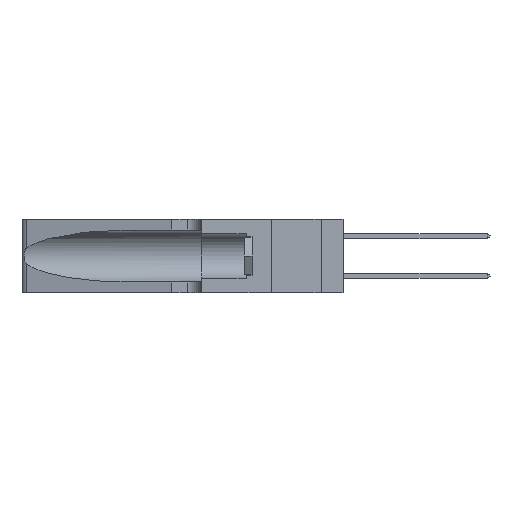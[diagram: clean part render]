
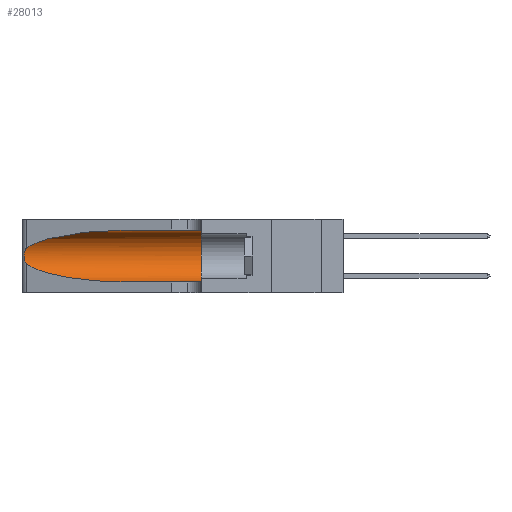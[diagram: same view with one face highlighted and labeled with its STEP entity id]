
A CAD part, left-side view. The second image highlights one B-rep face of the part: STEP entity #28013.
In plain terms, the highlighted cylindrical face has radius 3.308 mm (diameter 6.617 mm), a partial arc.
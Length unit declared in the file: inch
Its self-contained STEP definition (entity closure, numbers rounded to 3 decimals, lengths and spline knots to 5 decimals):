
#262 = VERTEX_POINT ( 'NONE', #25707 ) ;
#664 = CARTESIAN_POINT ( 'NONE',  ( 0.26075, 1.23896, 0.178 ) ) ;
#1474 = DIRECTION ( 'NONE',  ( 0., 0., 1. ) ) ;
#3393 = CARTESIAN_POINT ( 'NONE',  ( 0.25487, 1.22718, 0.14631 ) ) ;
#3429 = CARTESIAN_POINT ( 'NONE',  ( 0.25856, 1.23593, 0.16098 ) ) ;
#3610 = CARTESIAN_POINT ( 'NONE',  ( 0.1305, 0.35, 0.05475 ) ) ;
#3650 = DIRECTION ( 'NONE',  ( 0., -1., 0. ) ) ;
#3895 = CYLINDRICAL_SURFACE ( 'NONE', #28945, 0.13025 ) ;
#4145 = LINE ( 'NONE', #28352, #26777 ) ;
#4818 = CIRCLE ( 'NONE', #6387, 0.13025 ) ;
#5707 = VERTEX_POINT ( 'NONE', #3610 ) ;
#6070 = B_SPLINE_CURVE_WITH_KNOTS ( 'NONE', 3,
 ( #11568, #19654, #22416, #30575, #14310, #33290, #17061, #664, #19772, #3429, #22539, #6186, #25286, #8914 ),
 .UNSPECIFIED., .F., .F.,
 ( 4, 2, 2, 2, 2, 2, 4 ),
 ( 0., 0.00027, 0.00053, 0.00107, 0.0016, 0.00187, 0.00214 ),
 .UNSPECIFIED. ) ;
#6186 = CARTESIAN_POINT ( 'NONE',  ( 0.25639, 1.23186, 0.15144 ) ) ;
#6387 = AXIS2_PLACEMENT_3D ( 'NONE', #34087, #17839, #1474 ) ;
#7139 =( BOUNDED_CURVE ( )  B_SPLINE_CURVE ( 3, ( #25425, #30601, #30829, #14572 ),
 .UNSPECIFIED., .F., .F. ) 
 B_SPLINE_CURVE_WITH_KNOTS ( ( 4, 4 ),
 ( 1.5708, 2.84003 ),
 .UNSPECIFIED. ) 
 CURVE ( )  GEOMETRIC_REPRESENTATION_ITEM ( )  RATIONAL_B_SPLINE_CURVE ( ( 1., 0.87, 0.87, 1. ) ) 
 REPRESENTATION_ITEM ( '' )  );
#8318 = ORIENTED_EDGE ( 'NONE', *, *, #19628, .T. ) ;
#8880 = CARTESIAN_POINT ( 'NONE',  ( 0.1305, 0.72297, 0.05475 ) ) ;
#8914 = CARTESIAN_POINT ( 'NONE',  ( 0.25487, 1.22718, 0.14631 ) ) ;
#9402 = CARTESIAN_POINT ( 'NONE',  ( 0.1305, 0.72297, 0.05475 ) ) ;
#11568 = CARTESIAN_POINT ( 'NONE',  ( 0.25487, 1.22718, 0.22369 ) ) ;
#11782 = DIRECTION ( 'NONE',  ( 0., 0., -1. ) ) ;
#12039 = DIRECTION ( 'NONE',  ( 0., -1., 0. ) ) ;
#12633 = DIRECTION ( 'NONE',  ( 0., -1., 0. ) ) ;
#13146 = VERTEX_POINT ( 'NONE', #9402 ) ;
#14190 = CARTESIAN_POINT ( 'NONE',  ( 0.1305, 0.72297, 0.31525 ) ) ;
#14310 = CARTESIAN_POINT ( 'NONE',  ( 0.25854, 1.2359, 0.20912 ) ) ;
#14572 = CARTESIAN_POINT ( 'NONE',  ( 0.25487, 1.22718, 0.22369 ) ) ;
#15967 = EDGE_CURVE ( 'NONE', #31280, #22801, #6070, .T. ) ;
#16071 = EDGE_CURVE ( 'NONE', #18167, #262, #4145, .T. ) ;
#16887 = EDGE_CURVE ( 'NONE', #22801, #13146, #35047, .T. ) ;
#17061 = CARTESIAN_POINT ( 'NONE',  ( 0.26075, 1.23896, 0.19203 ) ) ;
#17433 = ORIENTED_EDGE ( 'NONE', *, *, #15967, .T. ) ;
#17839 = DIRECTION ( 'NONE',  ( 0., 1., 0. ) ) ;
#18167 = VERTEX_POINT ( 'NONE', #14190 ) ;
#19579 = ORIENTED_EDGE ( 'NONE', *, *, #16071, .F. ) ;
#19628 = EDGE_CURVE ( 'NONE', #13146, #5707, #25056, .T. ) ;
#19654 = CARTESIAN_POINT ( 'NONE',  ( 0.25555, 1.22994, 0.2215 ) ) ;
#19772 = CARTESIAN_POINT ( 'NONE',  ( 0.26017, 1.23833, 0.17102 ) ) ;
#22416 = CARTESIAN_POINT ( 'NONE',  ( 0.25639, 1.23184, 0.21858 ) ) ;
#22500 = CARTESIAN_POINT ( 'NONE',  ( 0.2373, 1.15595, 0.08982 ) ) ;
#22539 = CARTESIAN_POINT ( 'NONE',  ( 0.25789, 1.23486, 0.15765 ) ) ;
#22801 = VERTEX_POINT ( 'NONE', #34415 ) ;
#25056 = LINE ( 'NONE', #28941, #33042 ) ;
#25252 = CARTESIAN_POINT ( 'NONE',  ( 0.18966, 0.96281, 0.05475 ) ) ;
#25286 = CARTESIAN_POINT ( 'NONE',  ( 0.25555, 1.22993, 0.14849 ) ) ;
#25425 = CARTESIAN_POINT ( 'NONE',  ( 0.1305, 0.72297, 0.31525 ) ) ;
#25688 = FACE_OUTER_BOUND ( 'NONE', #26073, .T. ) ;
#25707 = CARTESIAN_POINT ( 'NONE',  ( 0.1305, 0.35, 0.31525 ) ) ;
#26073 = EDGE_LOOP ( 'NONE', ( #28708, #17433, #34225, #8318, #28130, #19579 ) ) ;
#26662 = CARTESIAN_POINT ( 'NONE',  ( 0.25487, 1.22718, 0.22369 ) ) ;
#26777 = VECTOR ( 'NONE', #12039, 39.37008 ) ;
#28013 = ADVANCED_FACE ( 'NONE', ( #25688 ), #3895, .F. ) ;
#28130 = ORIENTED_EDGE ( 'NONE', *, *, #31112, .F. ) ;
#28352 = CARTESIAN_POINT ( 'NONE',  ( 0.1305, 1.61858, 0.31525 ) ) ;
#28708 = ORIENTED_EDGE ( 'NONE', *, *, #34277, .T. ) ;
#28941 = CARTESIAN_POINT ( 'NONE',  ( 0.1305, 1.61858, 0.05475 ) ) ;
#28945 = AXIS2_PLACEMENT_3D ( 'NONE', #33509, #3650, #11782 ) ;
#30575 = CARTESIAN_POINT ( 'NONE',  ( 0.25787, 1.23484, 0.2124 ) ) ;
#30601 = CARTESIAN_POINT ( 'NONE',  ( 0.18966, 0.96281, 0.31525 ) ) ;
#30829 = CARTESIAN_POINT ( 'NONE',  ( 0.2373, 1.15595, 0.28018 ) ) ;
#31112 = EDGE_CURVE ( 'NONE', #262, #5707, #4818, .T. ) ;
#31280 = VERTEX_POINT ( 'NONE', #26662 ) ;
#33042 = VECTOR ( 'NONE', #12633, 39.37008 ) ;
#33290 = CARTESIAN_POINT ( 'NONE',  ( 0.26018, 1.23835, 0.19895 ) ) ;
#33509 = CARTESIAN_POINT ( 'NONE',  ( 0.1305, 1.61858, 0.185 ) ) ;
#34087 = CARTESIAN_POINT ( 'NONE',  ( 0.1305, 0.35, 0.185 ) ) ;
#34225 = ORIENTED_EDGE ( 'NONE', *, *, #16887, .T. ) ;
#34277 = EDGE_CURVE ( 'NONE', #18167, #31280, #7139, .T. ) ;
#34415 = CARTESIAN_POINT ( 'NONE',  ( 0.25487, 1.22718, 0.14631 ) ) ;
#35047 =( BOUNDED_CURVE ( )  B_SPLINE_CURVE ( 3, ( #3393, #22500, #25252, #8880 ),
 .UNSPECIFIED., .F., .F. ) 
 B_SPLINE_CURVE_WITH_KNOTS ( ( 4, 4 ),
 ( 3.44316, 4.71239 ),
 .UNSPECIFIED. ) 
 CURVE ( )  GEOMETRIC_REPRESENTATION_ITEM ( )  RATIONAL_B_SPLINE_CURVE ( ( 1., 0.87, 0.87, 1. ) ) 
 REPRESENTATION_ITEM ( '' )  );
